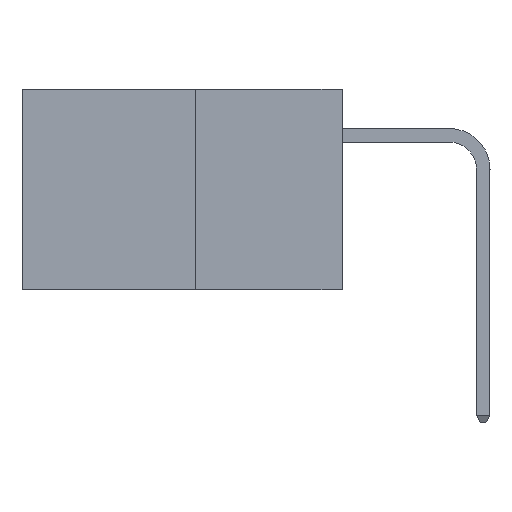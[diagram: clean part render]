
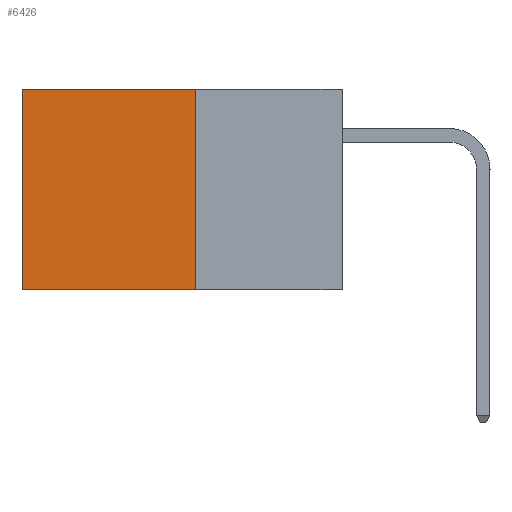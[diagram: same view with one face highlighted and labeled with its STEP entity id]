
A CAD part, left-side view. The second image highlights one B-rep face of the part: STEP entity #6426.
In plain terms, the highlighted planar face has unit normal (-1, 0, 0).
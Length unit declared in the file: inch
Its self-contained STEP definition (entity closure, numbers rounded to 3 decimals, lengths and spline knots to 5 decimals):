
#413 = CARTESIAN_POINT ( 'NONE',  ( 0.277, 0.27, -0.37 ) ) ;
#511 = FACE_OUTER_BOUND ( 'NONE', #1005, .T. ) ;
#626 = CARTESIAN_POINT ( 'NONE',  ( 0.277, 0.27, 0. ) ) ;
#662 = DIRECTION ( 'NONE',  ( 0., 1., 0. ) ) ;
#1005 = EDGE_LOOP ( 'NONE', ( #5424, #4985, #2812, #1346 ) ) ;
#1346 = ORIENTED_EDGE ( 'NONE', *, *, #11549, .T. ) ;
#2713 = EDGE_CURVE ( 'NONE', #5042, #12329, #12283, .T. ) ;
#2812 = ORIENTED_EDGE ( 'NONE', *, *, #9671, .F. ) ;
#2951 = CARTESIAN_POINT ( 'NONE',  ( 0.277, 0.27, -0.37 ) ) ;
#3525 = EDGE_CURVE ( 'NONE', #13868, #12329, #13633, .T. ) ;
#4089 = VECTOR ( 'NONE', #662, 39.37008 ) ;
#4268 = VECTOR ( 'NONE', #7066, 39.37008 ) ;
#4457 = LINE ( 'NONE', #6454, #4089 ) ;
#4985 = ORIENTED_EDGE ( 'NONE', *, *, #2713, .F. ) ;
#5042 = VERTEX_POINT ( 'NONE', #2951 ) ;
#5247 = PLANE ( 'NONE',  #9028 ) ;
#5424 = ORIENTED_EDGE ( 'NONE', *, *, #3525, .T. ) ;
#6282 = VECTOR ( 'NONE', #10177, 39.37008 ) ;
#6426 = ADVANCED_FACE ( 'NONE', ( #511 ), #5247, .F. ) ;
#6454 = CARTESIAN_POINT ( 'NONE',  ( 0.277, 0.27, 0. ) ) ;
#7066 = DIRECTION ( 'NONE',  ( 0., 0., -1. ) ) ;
#7317 = DIRECTION ( 'NONE',  ( 0., 0., -1. ) ) ;
#7545 = DIRECTION ( 'NONE',  ( 0., 0., -1. ) ) ;
#9028 = AXIS2_PLACEMENT_3D ( 'NONE', #13135, #14254, #7545 ) ;
#9060 = CARTESIAN_POINT ( 'NONE',  ( 0.277, 0.27, -0.37 ) ) ;
#9671 = EDGE_CURVE ( 'NONE', #12739, #5042, #9839, .T. ) ;
#9839 = LINE ( 'NONE', #413, #10524 ) ;
#10177 = DIRECTION ( 'NONE',  ( 0., 1., 0. ) ) ;
#10524 = VECTOR ( 'NONE', #7317, 39.37008 ) ;
#11549 = EDGE_CURVE ( 'NONE', #12739, #13868, #4457, .T. ) ;
#11813 = CARTESIAN_POINT ( 'NONE',  ( 0.277, 0.59, 0. ) ) ;
#12283 = LINE ( 'NONE', #9060, #6282 ) ;
#12329 = VERTEX_POINT ( 'NONE', #14527 ) ;
#12680 = CARTESIAN_POINT ( 'NONE',  ( 0.277, 0.59, -0.37 ) ) ;
#12739 = VERTEX_POINT ( 'NONE', #626 ) ;
#13135 = CARTESIAN_POINT ( 'NONE',  ( 0.277, 0.27, -0.37 ) ) ;
#13633 = LINE ( 'NONE', #12680, #4268 ) ;
#13868 = VERTEX_POINT ( 'NONE', #11813 ) ;
#14254 = DIRECTION ( 'NONE',  ( 1., 0., 0. ) ) ;
#14527 = CARTESIAN_POINT ( 'NONE',  ( 0.277, 0.59, -0.37 ) ) ;
